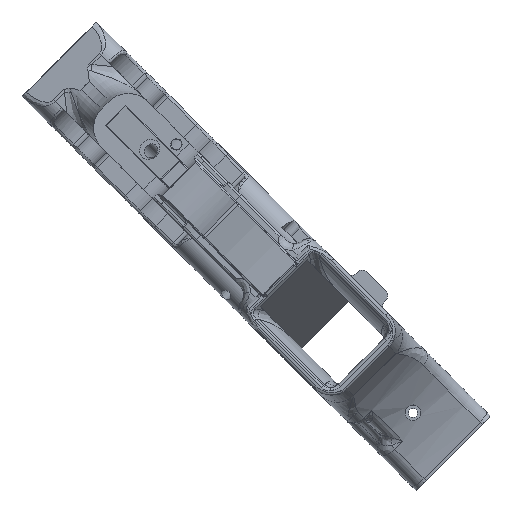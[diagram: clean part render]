
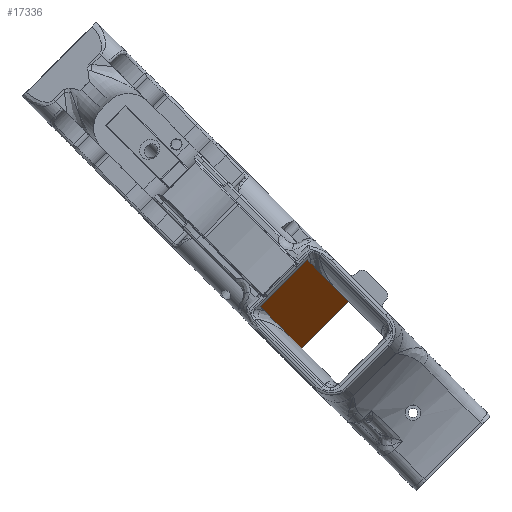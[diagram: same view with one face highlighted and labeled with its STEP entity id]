
A CAD part, top view. The second image highlights one B-rep face of the part: STEP entity #17336.
In plain terms, the highlighted planar face has unit normal (0.674, -0.674, 0.301).
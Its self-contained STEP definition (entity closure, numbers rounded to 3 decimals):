
#1188=PLANE('',#18623);
#2067=FACE_OUTER_BOUND('',#3048,.T.);
#3048=EDGE_LOOP('',(#15883,#15884,#15885,#15886));
#4612=LINE('',#27806,#6401);
#4657=LINE('',#28598,#6446);
#4688=LINE('',#29765,#6477);
#4692=LINE('',#29845,#6481);
#6401=VECTOR('',#21562,10.);
#6446=VECTOR('',#21739,10.);
#6477=VECTOR('',#21944,10.);
#6481=VECTOR('',#21966,10.);
#8288=VERTEX_POINT('',#27803);
#8289=VERTEX_POINT('',#27805);
#8366=VERTEX_POINT('',#28595);
#8367=VERTEX_POINT('',#28597);
#10454=EDGE_CURVE('',#8288,#8289,#4612,.T.);
#10570=EDGE_CURVE('',#8367,#8366,#4657,.T.);
#10685=EDGE_CURVE('',#8367,#8288,#4688,.T.);
#10695=EDGE_CURVE('',#8366,#8289,#4692,.T.);
#15883=ORIENTED_EDGE('',*,*,#10570,.T.);
#15884=ORIENTED_EDGE('',*,*,#10695,.T.);
#15885=ORIENTED_EDGE('',*,*,#10454,.F.);
#15886=ORIENTED_EDGE('',*,*,#10685,.F.);
#17336=ADVANCED_FACE('',(#2067),#1188,.F.);
#18623=AXIS2_PLACEMENT_3D('',#35829,#22875,#22876);
#21562=DIRECTION('',(-0.707,-0.707,0.));
#21739=DIRECTION('',(-0.707,-0.707,0.));
#21944=DIRECTION('',(0.213,-0.213,-0.954));
#21966=DIRECTION('',(0.213,-0.213,-0.954));
#22875=DIRECTION('center_axis',(-0.674,0.674,-0.301));
#22876=DIRECTION('ref_axis',(0.213,-0.213,-0.954));
#27803=CARTESIAN_POINT('',(106.823,102.221,125.1));
#27805=CARTESIAN_POINT('',(90.206,85.604,125.1));
#27806=CARTESIAN_POINT('',(141.63,137.028,125.1));
#28595=CARTESIAN_POINT('',(75.709,100.1,190.121));
#28597=CARTESIAN_POINT('',(92.326,116.717,190.121));
#28598=CARTESIAN_POINT('',(92.194,116.585,190.121));
#29765=CARTESIAN_POINT('',(85.754,123.29,219.602));
#29845=CARTESIAN_POINT('',(60.899,114.911,256.55));
#35829=CARTESIAN_POINT('Origin',(75.276,133.238,265.41));
